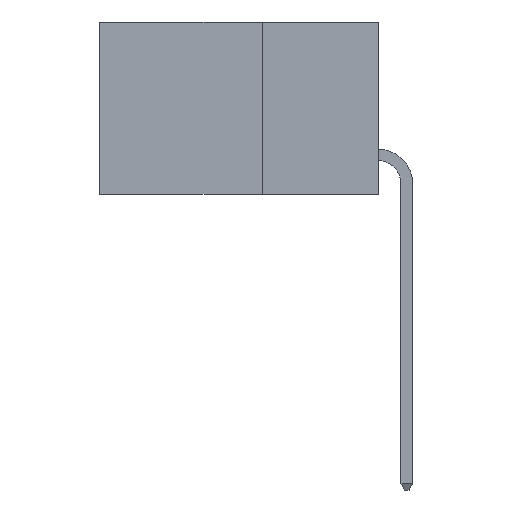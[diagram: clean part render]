
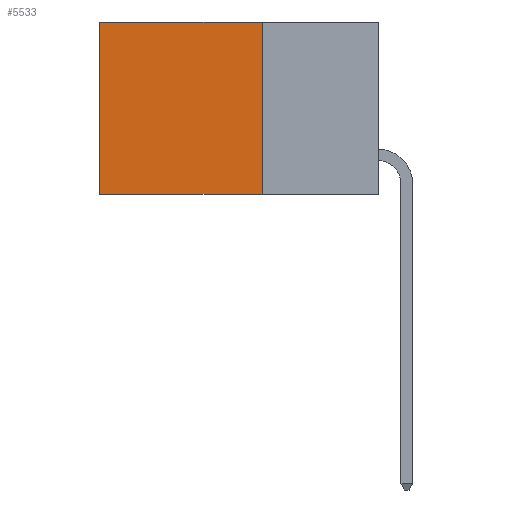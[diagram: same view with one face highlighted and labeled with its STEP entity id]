
A CAD part, left-side view. The second image highlights one B-rep face of the part: STEP entity #5533.
In plain terms, the highlighted planar face has unit normal (-1, 0, 0).
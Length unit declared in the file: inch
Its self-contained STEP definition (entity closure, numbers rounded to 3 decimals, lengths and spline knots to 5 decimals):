
#322 = LINE ( 'NONE', #414, #4625 ) ;
#358 = DIRECTION ( 'NONE',  ( 0., 1., 0. ) ) ;
#414 = CARTESIAN_POINT ( 'NONE',  ( 0.2615, 0.25, -0.37 ) ) ;
#953 = VERTEX_POINT ( 'NONE', #9155 ) ;
#1058 = PLANE ( 'NONE',  #5450 ) ;
#1386 = VECTOR ( 'NONE', #6864, 39.37008 ) ;
#1400 = VERTEX_POINT ( 'NONE', #3250 ) ;
#1808 = CARTESIAN_POINT ( 'NONE',  ( 0.2615, 0.6, -0.37 ) ) ;
#2705 = VERTEX_POINT ( 'NONE', #3830 ) ;
#2845 = DIRECTION ( 'NONE',  ( 0., 0., -1. ) ) ;
#3250 = CARTESIAN_POINT ( 'NONE',  ( 0.2615, 0.6, -0.37 ) ) ;
#3651 = CARTESIAN_POINT ( 'NONE',  ( 0.2615, 0.25, 0. ) ) ;
#3830 = CARTESIAN_POINT ( 'NONE',  ( 0.2615, 0.25, 0. ) ) ;
#3850 = EDGE_LOOP ( 'NONE', ( #5345, #8727, #9148, #8929 ) ) ;
#4369 = VECTOR ( 'NONE', #358, 39.37008 ) ;
#4383 = EDGE_CURVE ( 'NONE', #2705, #10225, #7563, .T. ) ;
#4625 = VECTOR ( 'NONE', #7155, 39.37008 ) ;
#4960 = EDGE_CURVE ( 'NONE', #953, #1400, #6309, .T. ) ;
#5345 = ORIENTED_EDGE ( 'NONE', *, *, #7472, .T. ) ;
#5450 = AXIS2_PLACEMENT_3D ( 'NONE', #6954, #7744, #2845 ) ;
#5533 = ADVANCED_FACE ( 'NONE', ( #10080 ), #1058, .F. ) ;
#6113 = DIRECTION ( 'NONE',  ( 0., 1., 0. ) ) ;
#6289 = CARTESIAN_POINT ( 'NONE',  ( 0.2615, 0.25, -0.37 ) ) ;
#6309 = LINE ( 'NONE', #6289, #4369 ) ;
#6552 = EDGE_CURVE ( 'NONE', #2705, #953, #322, .T. ) ;
#6864 = DIRECTION ( 'NONE',  ( 0., 0., -1. ) ) ;
#6954 = CARTESIAN_POINT ( 'NONE',  ( 0.2615, 0.25, -0.37 ) ) ;
#7155 = DIRECTION ( 'NONE',  ( 0., 0., -1. ) ) ;
#7472 = EDGE_CURVE ( 'NONE', #10225, #1400, #8255, .T. ) ;
#7563 = LINE ( 'NONE', #3651, #9363 ) ;
#7744 = DIRECTION ( 'NONE',  ( 1., 0., 0. ) ) ;
#8255 = LINE ( 'NONE', #1808, #1386 ) ;
#8727 = ORIENTED_EDGE ( 'NONE', *, *, #4960, .F. ) ;
#8929 = ORIENTED_EDGE ( 'NONE', *, *, #4383, .T. ) ;
#9148 = ORIENTED_EDGE ( 'NONE', *, *, #6552, .F. ) ;
#9155 = CARTESIAN_POINT ( 'NONE',  ( 0.2615, 0.25, -0.37 ) ) ;
#9363 = VECTOR ( 'NONE', #6113, 39.37008 ) ;
#10080 = FACE_OUTER_BOUND ( 'NONE', #3850, .T. ) ;
#10225 = VERTEX_POINT ( 'NONE', #10381 ) ;
#10381 = CARTESIAN_POINT ( 'NONE',  ( 0.2615, 0.6, 0. ) ) ;
